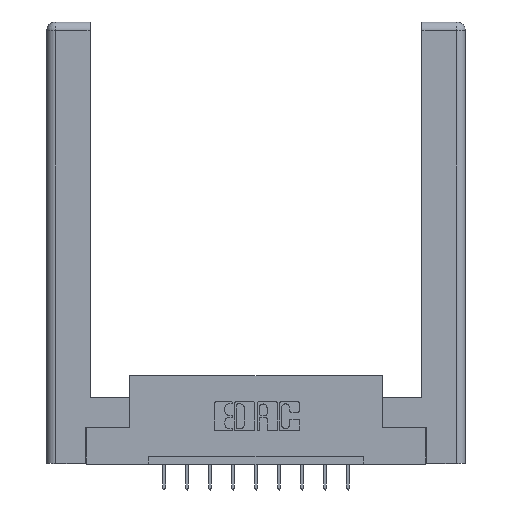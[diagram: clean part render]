
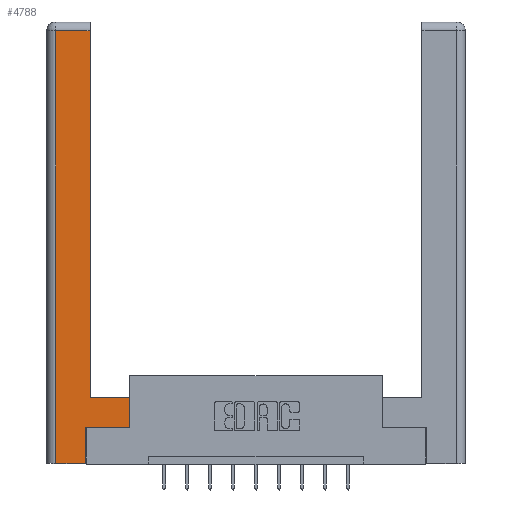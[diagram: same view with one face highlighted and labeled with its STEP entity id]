
A CAD part, top view. The second image highlights one B-rep face of the part: STEP entity #4788.
In plain terms, the highlighted planar face has unit normal (0, 0, 1).
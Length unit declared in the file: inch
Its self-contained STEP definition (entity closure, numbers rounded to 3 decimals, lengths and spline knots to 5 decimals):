
#226 = ORIENTED_EDGE ( 'NONE', *, *, #8461, .T. ) ;
#399 = VECTOR ( 'NONE', #11832, 39.37008 ) ;
#439 = CARTESIAN_POINT ( 'NONE',  ( 0.565, 0.245, 0. ) ) ;
#453 = CARTESIAN_POINT ( 'NONE',  ( 0.265, 0.245, 0. ) ) ;
#766 = EDGE_CURVE ( 'NONE', #2919, #9043, #9008, .T. ) ;
#966 = ORIENTED_EDGE ( 'NONE', *, *, #11196, .T. ) ;
#1216 = DIRECTION ( 'NONE',  ( 0., 1., 0. ) ) ;
#1273 = CARTESIAN_POINT ( 'NONE',  ( 0.295, 2.94, 0. ) ) ;
#1305 = DIRECTION ( 'NONE',  ( 0., 1., 0. ) ) ;
#1519 = LINE ( 'NONE', #7471, #4143 ) ;
#1541 = VERTEX_POINT ( 'NONE', #453 ) ;
#1738 = LINE ( 'NONE', #2504, #6674 ) ;
#1765 = DIRECTION ( 'NONE',  ( 0., 0., -1. ) ) ;
#2274 = DIRECTION ( 'NONE',  ( 1., 0., 0. ) ) ;
#2299 = VECTOR ( 'NONE', #2274, 39.37008 ) ;
#2504 = CARTESIAN_POINT ( 'NONE',  ( 0.565, 0.245, 0. ) ) ;
#2692 = CARTESIAN_POINT ( 'NONE',  ( 0.0615, 0., 0. ) ) ;
#2919 = VERTEX_POINT ( 'NONE', #10051 ) ;
#3092 = EDGE_CURVE ( 'NONE', #9043, #9552, #9103, .T. ) ;
#3774 = DIRECTION ( 'NONE',  ( -1., 0., 0. ) ) ;
#4143 = VECTOR ( 'NONE', #1216, 39.37008 ) ;
#4222 = ORIENTED_EDGE ( 'NONE', *, *, #13352, .T. ) ;
#4417 = EDGE_CURVE ( 'NONE', #9242, #1541, #1519, .T. ) ;
#4788 = ADVANCED_FACE ( 'NONE', ( #5933 ), #10235, .F. ) ;
#5016 = CARTESIAN_POINT ( 'NONE',  ( 0.295, 0.45, 0. ) ) ;
#5933 = FACE_OUTER_BOUND ( 'NONE', #7918, .T. ) ;
#5980 = ORIENTED_EDGE ( 'NONE', *, *, #766, .T. ) ;
#6340 = VERTEX_POINT ( 'NONE', #12555 ) ;
#6453 = VERTEX_POINT ( 'NONE', #11501 ) ;
#6467 = CARTESIAN_POINT ( 'NONE',  ( 0.0615, 2.94, 0. ) ) ;
#6636 = DIRECTION ( 'NONE',  ( 0., 1., 0. ) ) ;
#6674 = VECTOR ( 'NONE', #7792, 39.37008 ) ;
#6737 = CARTESIAN_POINT ( 'NONE',  ( 0.565, 0.45, 0. ) ) ;
#7353 = EDGE_CURVE ( 'NONE', #9198, #2919, #8697, .T. ) ;
#7471 = CARTESIAN_POINT ( 'NONE',  ( 0.265, 0.245, 0. ) ) ;
#7548 = LINE ( 'NONE', #2692, #13341 ) ;
#7774 = VECTOR ( 'NONE', #6636, 39.37008 ) ;
#7792 = DIRECTION ( 'NONE',  ( 1., 0., 0. ) ) ;
#7918 = EDGE_LOOP ( 'NONE', ( #10945, #226, #10624, #966, #8550, #4222, #13514, #5980 ) ) ;
#8210 = CARTESIAN_POINT ( 'NONE',  ( 0., 0., 0. ) ) ;
#8286 = CARTESIAN_POINT ( 'NONE',  ( 0.265, 0., 0. ) ) ;
#8461 = EDGE_CURVE ( 'NONE', #9552, #6340, #12448, .T. ) ;
#8550 = ORIENTED_EDGE ( 'NONE', *, *, #4417, .T. ) ;
#8613 = CARTESIAN_POINT ( 'NONE',  ( 0.295, 3., 0. ) ) ;
#8697 = LINE ( 'NONE', #6737, #12328 ) ;
#9008 = LINE ( 'NONE', #5016, #9337 ) ;
#9043 = VERTEX_POINT ( 'NONE', #9872 ) ;
#9103 = LINE ( 'NONE', #8613, #7774 ) ;
#9198 = VERTEX_POINT ( 'NONE', #439 ) ;
#9242 = VERTEX_POINT ( 'NONE', #8286 ) ;
#9337 = VECTOR ( 'NONE', #12393, 39.37008 ) ;
#9552 = VERTEX_POINT ( 'NONE', #1273 ) ;
#9872 = CARTESIAN_POINT ( 'NONE',  ( 0.295, 0.45, 0. ) ) ;
#10051 = CARTESIAN_POINT ( 'NONE',  ( 0.565, 0.45, 0. ) ) ;
#10235 = PLANE ( 'NONE',  #11738 ) ;
#10531 = CARTESIAN_POINT ( 'NONE',  ( 0.265, 0., 0. ) ) ;
#10541 = LINE ( 'NONE', #10531, #2299 ) ;
#10624 = ORIENTED_EDGE ( 'NONE', *, *, #11890, .T. ) ;
#10945 = ORIENTED_EDGE ( 'NONE', *, *, #3092, .T. ) ;
#11078 = DIRECTION ( 'NONE',  ( 0., -1., 0. ) ) ;
#11196 = EDGE_CURVE ( 'NONE', #6453, #9242, #10541, .T. ) ;
#11501 = CARTESIAN_POINT ( 'NONE',  ( 0.0615, 0., 0. ) ) ;
#11738 = AXIS2_PLACEMENT_3D ( 'NONE', #8210, #1765, #3774 ) ;
#11832 = DIRECTION ( 'NONE',  ( -1., 0., 0. ) ) ;
#11890 = EDGE_CURVE ( 'NONE', #6340, #6453, #7548, .T. ) ;
#12328 = VECTOR ( 'NONE', #1305, 39.37008 ) ;
#12393 = DIRECTION ( 'NONE',  ( -1., 0., 0. ) ) ;
#12448 = LINE ( 'NONE', #6467, #399 ) ;
#12555 = CARTESIAN_POINT ( 'NONE',  ( 0.0615, 2.94, 0. ) ) ;
#13341 = VECTOR ( 'NONE', #11078, 39.37008 ) ;
#13352 = EDGE_CURVE ( 'NONE', #1541, #9198, #1738, .T. ) ;
#13514 = ORIENTED_EDGE ( 'NONE', *, *, #7353, .T. ) ;
